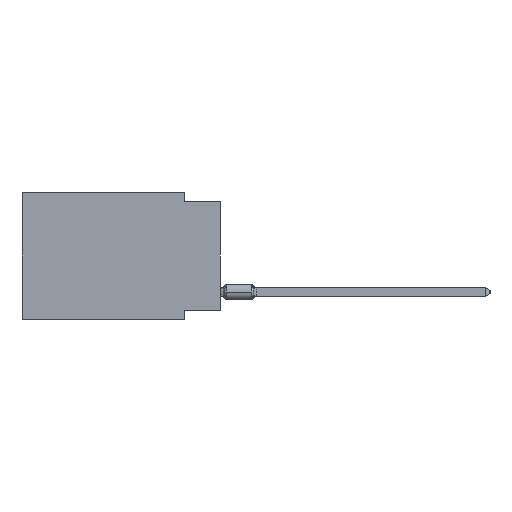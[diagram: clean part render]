
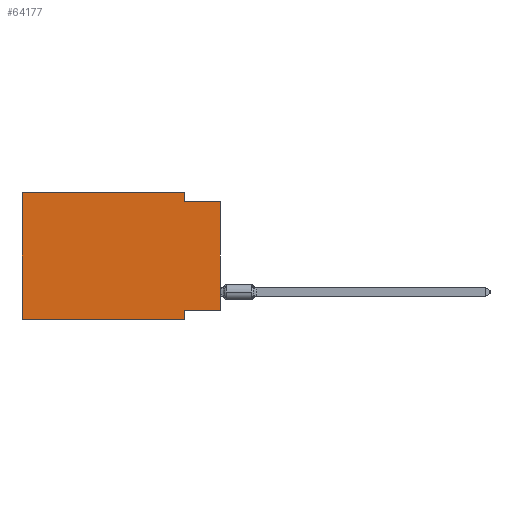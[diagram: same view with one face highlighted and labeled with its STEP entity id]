
A CAD part, left-side view. The second image highlights one B-rep face of the part: STEP entity #64177.
In plain terms, the highlighted planar face has unit normal (-1, 0, 0).
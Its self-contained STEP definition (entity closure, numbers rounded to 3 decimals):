
#88 = LINE ( 'NONE', #55831, #33552 ) ;
#2227 = LINE ( 'NONE', #51793, #22605 ) ;
#2230 = ORIENTED_EDGE ( 'NONE', *, *, #35913, .F. ) ;
#2899 = VERTEX_POINT ( 'NONE', #59119 ) ;
#4870 = VERTEX_POINT ( 'NONE', #41333 ) ;
#5580 = CARTESIAN_POINT ( 'NONE',  ( 0., 0., -0.635 ) ) ;
#5907 = DIRECTION ( 'NONE',  ( 0., -1., 0. ) ) ;
#7511 = ORIENTED_EDGE ( 'NONE', *, *, #63337, .T. ) ;
#8910 = DIRECTION ( 'NONE',  ( 0., 0., 1. ) ) ;
#10477 = LINE ( 'NONE', #44089, #59945 ) ;
#10691 = FACE_OUTER_BOUND ( 'NONE', #63326, .T. ) ;
#11025 = EDGE_CURVE ( 'NONE', #60015, #29585, #18456, .T. ) ;
#12919 = DIRECTION ( 'NONE',  ( 0., 1., 0. ) ) ;
#13626 = ORIENTED_EDGE ( 'NONE', *, *, #30328, .F. ) ;
#14632 = PLANE ( 'NONE',  #17608 ) ;
#16191 = ORIENTED_EDGE ( 'NONE', *, *, #28269, .F. ) ;
#17608 = AXIS2_PLACEMENT_3D ( 'NONE', #29957, #46789, #36700 ) ;
#17758 = CARTESIAN_POINT ( 'NONE',  ( 0., 13.97, -8.89 ) ) ;
#17793 = CARTESIAN_POINT ( 'NONE',  ( 0., 2.54, -8.89 ) ) ;
#17804 = LINE ( 'NONE', #57581, #42672 ) ;
#18456 = LINE ( 'NONE', #17793, #19803 ) ;
#18992 = CARTESIAN_POINT ( 'NONE',  ( 0., 0., -8.255 ) ) ;
#19643 = VECTOR ( 'NONE', #24257, 1000. ) ;
#19803 = VECTOR ( 'NONE', #42916, 1000. ) ;
#21241 = LINE ( 'NONE', #5580, #54085 ) ;
#22605 = VECTOR ( 'NONE', #37137, 1000. ) ;
#24257 = DIRECTION ( 'NONE',  ( 0., 0., 1. ) ) ;
#25407 = EDGE_CURVE ( 'NONE', #36852, #2899, #10477, .T. ) ;
#26180 = CARTESIAN_POINT ( 'NONE',  ( 0., 2.54, -8.255 ) ) ;
#28269 = EDGE_CURVE ( 'NONE', #2899, #44176, #2227, .T. ) ;
#28712 = CARTESIAN_POINT ( 'NONE',  ( 0., 2.54, -8.89 ) ) ;
#29585 = VERTEX_POINT ( 'NONE', #28712 ) ;
#29957 = CARTESIAN_POINT ( 'NONE',  ( 0., 13.97, 0. ) ) ;
#30328 = EDGE_CURVE ( 'NONE', #44176, #4870, #21241, .T. ) ;
#31371 = DIRECTION ( 'NONE',  ( 0., -1., 0. ) ) ;
#31437 = VERTEX_POINT ( 'NONE', #18992 ) ;
#33262 = ORIENTED_EDGE ( 'NONE', *, *, #25407, .F. ) ;
#33552 = VECTOR ( 'NONE', #31371, 1000. ) ;
#35913 = EDGE_CURVE ( 'NONE', #44163, #36852, #44120, .T. ) ;
#36041 = CARTESIAN_POINT ( 'NONE',  ( 0., 13.97, 0. ) ) ;
#36700 = DIRECTION ( 'NONE',  ( 0., 0., -1. ) ) ;
#36852 = VERTEX_POINT ( 'NONE', #36041 ) ;
#37137 = DIRECTION ( 'NONE',  ( 0., 0., -1. ) ) ;
#37452 = ORIENTED_EDGE ( 'NONE', *, *, #11025, .F. ) ;
#38909 = CARTESIAN_POINT ( 'NONE',  ( 0., 13.97, 0. ) ) ;
#41333 = CARTESIAN_POINT ( 'NONE',  ( 0., 0., -0.635 ) ) ;
#42672 = VECTOR ( 'NONE', #12919, 1000. ) ;
#42916 = DIRECTION ( 'NONE',  ( 0., 0., -1. ) ) ;
#44089 = CARTESIAN_POINT ( 'NONE',  ( 0., 13.97, 0. ) ) ;
#44120 = LINE ( 'NONE', #38909, #47926 ) ;
#44163 = VERTEX_POINT ( 'NONE', #17758 ) ;
#44176 = VERTEX_POINT ( 'NONE', #52648 ) ;
#46789 = DIRECTION ( 'NONE',  ( 1., 0., 0. ) ) ;
#47926 = VECTOR ( 'NONE', #8910, 1000. ) ;
#48309 = ORIENTED_EDGE ( 'NONE', *, *, #53825, .T. ) ;
#49031 = CARTESIAN_POINT ( 'NONE',  ( 0., 0., 0. ) ) ;
#49968 = ORIENTED_EDGE ( 'NONE', *, *, #58279, .F. ) ;
#51793 = CARTESIAN_POINT ( 'NONE',  ( 0., 2.54, 0. ) ) ;
#52648 = CARTESIAN_POINT ( 'NONE',  ( 0., 2.54, -0.635 ) ) ;
#53825 = EDGE_CURVE ( 'NONE', #44163, #29585, #88, .T. ) ;
#54085 = VECTOR ( 'NONE', #5907, 1000. ) ;
#55831 = CARTESIAN_POINT ( 'NONE',  ( 0., 13.97, -8.89 ) ) ;
#57581 = CARTESIAN_POINT ( 'NONE',  ( 0., 0., -8.255 ) ) ;
#58279 = EDGE_CURVE ( 'NONE', #31437, #60015, #17804, .T. ) ;
#59119 = CARTESIAN_POINT ( 'NONE',  ( 0., 2.54, 0. ) ) ;
#59125 = LINE ( 'NONE', #49031, #19643 ) ;
#59945 = VECTOR ( 'NONE', #64286, 1000. ) ;
#60015 = VERTEX_POINT ( 'NONE', #26180 ) ;
#63326 = EDGE_LOOP ( 'NONE', ( #7511, #13626, #16191, #33262, #2230, #48309, #37452, #49968 ) ) ;
#63337 = EDGE_CURVE ( 'NONE', #31437, #4870, #59125, .T. ) ;
#64177 = ADVANCED_FACE ( 'NONE', ( #10691 ), #14632, .F. ) ;
#64286 = DIRECTION ( 'NONE',  ( 0., -1., 0. ) ) ;
